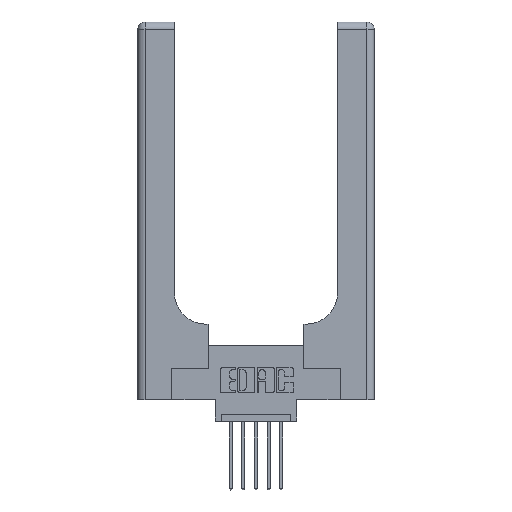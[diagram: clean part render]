
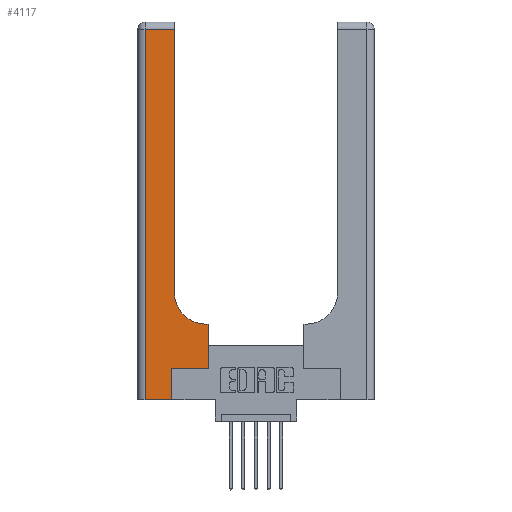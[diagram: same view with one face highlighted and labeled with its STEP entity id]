
A CAD part, top view. The second image highlights one B-rep face of the part: STEP entity #4117.
In plain terms, the highlighted planar face has unit normal (0, 0, 1).
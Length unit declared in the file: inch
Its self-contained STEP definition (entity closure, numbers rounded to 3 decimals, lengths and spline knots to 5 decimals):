
#241 = CARTESIAN_POINT ( 'NONE',  ( 0.269, 0., 0.37 ) ) ;
#407 = CARTESIAN_POINT ( 'NONE',  ( 0., 3., 0.37 ) ) ;
#653 = VECTOR ( 'NONE', #5168, 39.37008 ) ;
#809 = CARTESIAN_POINT ( 'NONE',  ( 0., 0., 0.37 ) ) ;
#1840 = LINE ( 'NONE', #809, #653 ) ;
#1901 = CARTESIAN_POINT ( 'NONE',  ( 0.269, 0., 0.37 ) ) ;
#1921 = CARTESIAN_POINT ( 'NONE',  ( 0.06, 3., 0.37 ) ) ;
#2020 = ORIENTED_EDGE ( 'NONE', *, *, #12865, .T. ) ;
#2431 = AXIS2_PLACEMENT_3D ( 'NONE', #12501, #6012, #10313 ) ;
#2892 = CARTESIAN_POINT ( 'NONE',  ( 0.5585, 0.6, 0.37 ) ) ;
#3036 = DIRECTION ( 'NONE',  ( -1., 0., 0. ) ) ;
#3093 = CARTESIAN_POINT ( 'NONE',  ( 0.2915, 0.6, 0.37 ) ) ;
#3821 = ORIENTED_EDGE ( 'NONE', *, *, #11446, .T. ) ;
#3834 = CARTESIAN_POINT ( 'NONE',  ( 0.06, 0., 0.37 ) ) ;
#4109 = CARTESIAN_POINT ( 'NONE',  ( 0.5415, 0.6, 0.37 ) ) ;
#4117 = ADVANCED_FACE ( 'NONE', ( #8121 ), #13755, .F. ) ;
#4199 = EDGE_CURVE ( 'NONE', #11924, #7109, #6764, .T. ) ;
#4211 = ORIENTED_EDGE ( 'NONE', *, *, #9905, .T. ) ;
#4220 = EDGE_CURVE ( 'NONE', #9323, #5531, #7100, .T. ) ;
#4668 = CIRCLE ( 'NONE', #2431, 0.25 ) ;
#4793 = VECTOR ( 'NONE', #5304, 39.37008 ) ;
#4919 = VECTOR ( 'NONE', #12935, 39.37008 ) ;
#5040 = EDGE_CURVE ( 'NONE', #5531, #5740, #1840, .T. ) ;
#5168 = DIRECTION ( 'NONE',  ( 1., 0., 0. ) ) ;
#5304 = DIRECTION ( 'NONE',  ( 0., 1., 0. ) ) ;
#5531 = VERTEX_POINT ( 'NONE', #3834 ) ;
#5740 = VERTEX_POINT ( 'NONE', #241 ) ;
#5835 = CARTESIAN_POINT ( 'NONE',  ( 0.2915, 3., 0.37 ) ) ;
#5848 = DIRECTION ( 'NONE',  ( 1., 0., 0. ) ) ;
#5936 = AXIS2_PLACEMENT_3D ( 'NONE', #407, #10544, #3036 ) ;
#5961 = ORIENTED_EDGE ( 'NONE', *, *, #4199, .T. ) ;
#6012 = DIRECTION ( 'NONE',  ( 0., 0., -1. ) ) ;
#6043 = ORIENTED_EDGE ( 'NONE', *, *, #5040, .T. ) ;
#6269 = CARTESIAN_POINT ( 'NONE',  ( 0.5585, 0.25, 0.37 ) ) ;
#6304 = VERTEX_POINT ( 'NONE', #11922 ) ;
#6400 = DIRECTION ( 'NONE',  ( 0., -1., 0. ) ) ;
#6508 = LINE ( 'NONE', #1901, #6860 ) ;
#6764 = LINE ( 'NONE', #3093, #4919 ) ;
#6800 = LINE ( 'NONE', #8472, #4793 ) ;
#6860 = VECTOR ( 'NONE', #11744, 39.37008 ) ;
#6927 = CARTESIAN_POINT ( 'NONE',  ( 0.269, 0.25, 0.37 ) ) ;
#7094 = EDGE_LOOP ( 'NONE', ( #8223, #13528, #10768, #6043, #8347, #2020, #3821, #5961, #4211 ) ) ;
#7100 = LINE ( 'NONE', #1921, #10695 ) ;
#7109 = VERTEX_POINT ( 'NONE', #4109 ) ;
#7360 = VECTOR ( 'NONE', #11406, 39.37008 ) ;
#7421 = VERTEX_POINT ( 'NONE', #12470 ) ;
#8121 = FACE_OUTER_BOUND ( 'NONE', #7094, .T. ) ;
#8223 = ORIENTED_EDGE ( 'NONE', *, *, #9407, .T. ) ;
#8347 = ORIENTED_EDGE ( 'NONE', *, *, #9485, .T. ) ;
#8472 = CARTESIAN_POINT ( 'NONE',  ( 0.5585, 0.25, 0.37 ) ) ;
#8697 = VECTOR ( 'NONE', #5848, 39.37008 ) ;
#9323 = VERTEX_POINT ( 'NONE', #11378 ) ;
#9405 = LINE ( 'NONE', #6927, #8697 ) ;
#9407 = EDGE_CURVE ( 'NONE', #6304, #14046, #10804, .T. ) ;
#9485 = EDGE_CURVE ( 'NONE', #5740, #7421, #6508, .T. ) ;
#9878 = EDGE_CURVE ( 'NONE', #14046, #9323, #10471, .T. ) ;
#9905 = EDGE_CURVE ( 'NONE', #7109, #6304, #4668, .T. ) ;
#10313 = DIRECTION ( 'NONE',  ( 1., 0., 0. ) ) ;
#10471 = LINE ( 'NONE', #11311, #7360 ) ;
#10544 = DIRECTION ( 'NONE',  ( 0., 0., -1. ) ) ;
#10662 = VERTEX_POINT ( 'NONE', #6269 ) ;
#10695 = VECTOR ( 'NONE', #6400, 39.37008 ) ;
#10768 = ORIENTED_EDGE ( 'NONE', *, *, #4220, .T. ) ;
#10804 = LINE ( 'NONE', #5835, #12681 ) ;
#11311 = CARTESIAN_POINT ( 'NONE',  ( 0., 2.94, 0.37 ) ) ;
#11378 = CARTESIAN_POINT ( 'NONE',  ( 0.06, 2.94, 0.37 ) ) ;
#11406 = DIRECTION ( 'NONE',  ( -1., 0., 0. ) ) ;
#11446 = EDGE_CURVE ( 'NONE', #10662, #11924, #6800, .T. ) ;
#11651 = DIRECTION ( 'NONE',  ( 0., 1., 0. ) ) ;
#11744 = DIRECTION ( 'NONE',  ( 0., 1., 0. ) ) ;
#11922 = CARTESIAN_POINT ( 'NONE',  ( 0.2915, 0.85, 0.37 ) ) ;
#11924 = VERTEX_POINT ( 'NONE', #2892 ) ;
#12372 = CARTESIAN_POINT ( 'NONE',  ( 0.2915, 2.94, 0.37 ) ) ;
#12470 = CARTESIAN_POINT ( 'NONE',  ( 0.269, 0.25, 0.37 ) ) ;
#12501 = CARTESIAN_POINT ( 'NONE',  ( 0.5415, 0.85, 0.37 ) ) ;
#12681 = VECTOR ( 'NONE', #11651, 39.37008 ) ;
#12865 = EDGE_CURVE ( 'NONE', #7421, #10662, #9405, .T. ) ;
#12935 = DIRECTION ( 'NONE',  ( -1., 0., 0. ) ) ;
#13528 = ORIENTED_EDGE ( 'NONE', *, *, #9878, .T. ) ;
#13755 = PLANE ( 'NONE',  #5936 ) ;
#14046 = VERTEX_POINT ( 'NONE', #12372 ) ;
